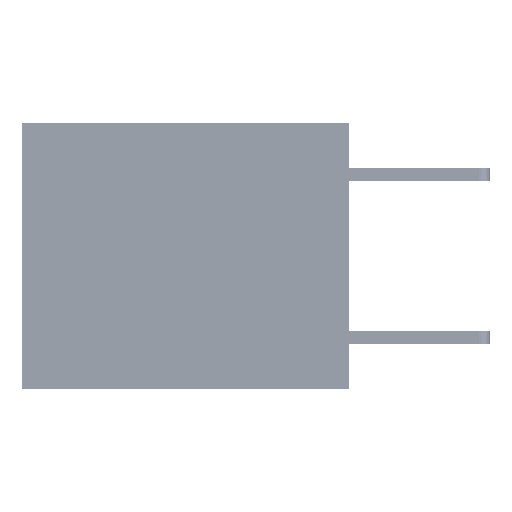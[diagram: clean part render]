
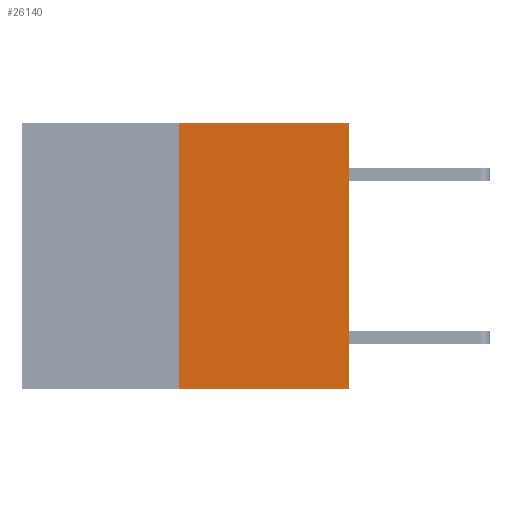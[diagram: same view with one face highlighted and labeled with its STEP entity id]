
A CAD part, left-side view. The second image highlights one B-rep face of the part: STEP entity #26140.
In plain terms, the highlighted planar face has unit normal (-1, 0, 0).
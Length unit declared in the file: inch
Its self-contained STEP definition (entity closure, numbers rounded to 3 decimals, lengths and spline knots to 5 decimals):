
#865 = VECTOR ( 'NONE', #18266, 39.37008 ) ;
#2231 = VECTOR ( 'NONE', #34533, 39.37008 ) ;
#3044 = VERTEX_POINT ( 'NONE', #28587 ) ;
#4850 = ORIENTED_EDGE ( 'NONE', *, *, #17721, .T. ) ;
#5373 = PLANE ( 'NONE',  #6687 ) ;
#5461 = LINE ( 'NONE', #31612, #8168 ) ;
#6154 = FACE_OUTER_BOUND ( 'NONE', #16150, .T. ) ;
#6687 = AXIS2_PLACEMENT_3D ( 'NONE', #16809, #36468, #25478 ) ;
#6716 = EDGE_CURVE ( 'NONE', #3044, #28377, #26840, .T. ) ;
#8168 = VECTOR ( 'NONE', #23370, 39.37008 ) ;
#8384 = LINE ( 'NONE', #35411, #865 ) ;
#8641 = VERTEX_POINT ( 'NONE', #29995 ) ;
#8673 = VERTEX_POINT ( 'NONE', #15714 ) ;
#9428 = DIRECTION ( 'NONE',  ( 0., -1., 0. ) ) ;
#12033 = EDGE_CURVE ( 'NONE', #8641, #8673, #5461, .T. ) ;
#15590 = ORIENTED_EDGE ( 'NONE', *, *, #26041, .F. ) ;
#15714 = CARTESIAN_POINT ( 'NONE',  ( 0., 0., 0. ) ) ;
#16150 = EDGE_LOOP ( 'NONE', ( #31728, #4850, #30418, #15590 ) ) ;
#16809 = CARTESIAN_POINT ( 'NONE',  ( 0., 0.6, 0. ) ) ;
#17721 = EDGE_CURVE ( 'NONE', #3044, #8641, #22424, .T. ) ;
#18266 = DIRECTION ( 'NONE',  ( 0., -1., 0. ) ) ;
#21060 = CARTESIAN_POINT ( 'NONE',  ( 0., 0.312, 0. ) ) ;
#22018 = VECTOR ( 'NONE', #9428, 39.37008 ) ;
#22424 = LINE ( 'NONE', #23679, #22018 ) ;
#23370 = DIRECTION ( 'NONE',  ( 0., 0., 1. ) ) ;
#23679 = CARTESIAN_POINT ( 'NONE',  ( 0., 0.6, -0.49 ) ) ;
#25478 = DIRECTION ( 'NONE',  ( 0., 0., -1. ) ) ;
#26041 = EDGE_CURVE ( 'NONE', #28377, #8673, #8384, .T. ) ;
#26140 = ADVANCED_FACE ( 'NONE', ( #6154 ), #5373, .F. ) ;
#26840 = LINE ( 'NONE', #36669, #2231 ) ;
#28377 = VERTEX_POINT ( 'NONE', #21060 ) ;
#28587 = CARTESIAN_POINT ( 'NONE',  ( 0., 0.312, -0.49 ) ) ;
#29995 = CARTESIAN_POINT ( 'NONE',  ( 0., 0., -0.49 ) ) ;
#30418 = ORIENTED_EDGE ( 'NONE', *, *, #12033, .T. ) ;
#31612 = CARTESIAN_POINT ( 'NONE',  ( 0., 0., 0. ) ) ;
#31728 = ORIENTED_EDGE ( 'NONE', *, *, #6716, .F. ) ;
#34533 = DIRECTION ( 'NONE',  ( 0., 0., 1. ) ) ;
#35411 = CARTESIAN_POINT ( 'NONE',  ( 0., 0.6, 0. ) ) ;
#36468 = DIRECTION ( 'NONE',  ( 1., 0., 0. ) ) ;
#36669 = CARTESIAN_POINT ( 'NONE',  ( 0., 0.312, -0.49 ) ) ;
